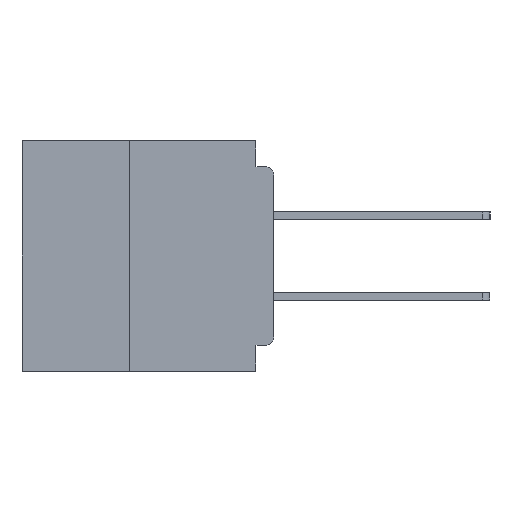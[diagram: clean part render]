
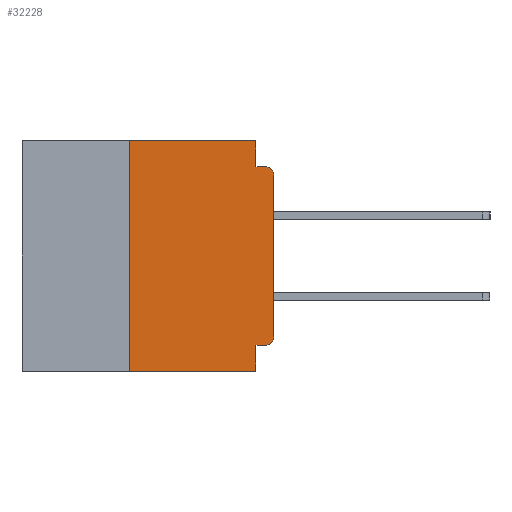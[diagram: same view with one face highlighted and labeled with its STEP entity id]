
A CAD part, left-side view. The second image highlights one B-rep face of the part: STEP entity #32228.
In plain terms, the highlighted planar face has unit normal (-1, 0, 0).
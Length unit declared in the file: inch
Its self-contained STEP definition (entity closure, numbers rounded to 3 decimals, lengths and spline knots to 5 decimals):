
#63 = CARTESIAN_POINT ( 'NONE',  ( 0., 0.031, -0.4 ) ) ;
#301 = FACE_OUTER_BOUND ( 'NONE', #5033, .T. ) ;
#354 = DIRECTION ( 'NONE',  ( 0., 0., -1. ) ) ;
#1073 = EDGE_CURVE ( 'NONE', #8097, #22778, #32696, .T. ) ;
#1078 = CARTESIAN_POINT ( 'NONE',  ( 0., 0.25, 0. ) ) ;
#1639 = LINE ( 'NONE', #37122, #17324 ) ;
#2381 = EDGE_CURVE ( 'NONE', #8097, #33023, #16201, .T. ) ;
#3934 = ORIENTED_EDGE ( 'NONE', *, *, #2381, .T. ) ;
#4353 = EDGE_CURVE ( 'NONE', #19786, #31630, #17419, .T. ) ;
#4840 = VERTEX_POINT ( 'NONE', #6198 ) ;
#4859 = CARTESIAN_POINT ( 'NONE',  ( 0., 0.031, 0. ) ) ;
#5033 = EDGE_LOOP ( 'NONE', ( #5572, #15043, #29890, #26032, #13446, #22626, #3934, #21858, #25732, #12016 ) ) ;
#5572 = ORIENTED_EDGE ( 'NONE', *, *, #6417, .T. ) ;
#5664 = VERTEX_POINT ( 'NONE', #15460 ) ;
#6160 = VECTOR ( 'NONE', #27031, 39.37008 ) ;
#6183 = CARTESIAN_POINT ( 'NONE',  ( 0., 0.015, -0.355 ) ) ;
#6198 = CARTESIAN_POINT ( 'NONE',  ( 0., 0., -0.34 ) ) ;
#6417 = EDGE_CURVE ( 'NONE', #4840, #19786, #29302, .T. ) ;
#8097 = VERTEX_POINT ( 'NONE', #29128 ) ;
#8337 = CARTESIAN_POINT ( 'NONE',  ( 0., 0., -0.045 ) ) ;
#9263 = VECTOR ( 'NONE', #20556, 39.37008 ) ;
#10635 = AXIS2_PLACEMENT_3D ( 'NONE', #28412, #11251, #31383 ) ;
#10794 = DIRECTION ( 'NONE',  ( 0., 0., -1. ) ) ;
#11016 = CARTESIAN_POINT ( 'NONE',  ( 0., 0.031, 0. ) ) ;
#11251 = DIRECTION ( 'NONE',  ( 1., 0., 0. ) ) ;
#11285 = VECTOR ( 'NONE', #16292, 39.37008 ) ;
#12016 = ORIENTED_EDGE ( 'NONE', *, *, #26692, .T. ) ;
#13446 = ORIENTED_EDGE ( 'NONE', *, *, #28144, .F. ) ;
#14056 = PLANE ( 'NONE',  #10635 ) ;
#14420 = LINE ( 'NONE', #8337, #15321 ) ;
#14427 = VECTOR ( 'NONE', #10794, 39.37008 ) ;
#14784 = EDGE_CURVE ( 'NONE', #24814, #5664, #37004, .T. ) ;
#15043 = ORIENTED_EDGE ( 'NONE', *, *, #4353, .T. ) ;
#15321 = VECTOR ( 'NONE', #34233, 39.37008 ) ;
#15460 = CARTESIAN_POINT ( 'NONE',  ( 0., 0.031, -0.045 ) ) ;
#15681 = CARTESIAN_POINT ( 'NONE',  ( 0., 0., -0.06 ) ) ;
#16118 = AXIS2_PLACEMENT_3D ( 'NONE', #17926, #17888, #17855 ) ;
#16201 = LINE ( 'NONE', #20604, #9263 ) ;
#16292 = DIRECTION ( 'NONE',  ( 0., -1., 0. ) ) ;
#17324 = VECTOR ( 'NONE', #20376, 39.37008 ) ;
#17419 = CIRCLE ( 'NONE', #16118, 0.015 ) ;
#17543 = CARTESIAN_POINT ( 'NONE',  ( 0., 0.031, -0.355 ) ) ;
#17855 = DIRECTION ( 'NONE',  ( 0., 0., -1. ) ) ;
#17888 = DIRECTION ( 'NONE',  ( -1., 0., 0. ) ) ;
#17926 = CARTESIAN_POINT ( 'NONE',  ( 0., 0.015, -0.06 ) ) ;
#18024 = DIRECTION ( 'NONE',  ( -1., 0., 0. ) ) ;
#19013 = EDGE_CURVE ( 'NONE', #5664, #31630, #14420, .T. ) ;
#19786 = VERTEX_POINT ( 'NONE', #15681 ) ;
#20376 = DIRECTION ( 'NONE',  ( 0., 1., 0. ) ) ;
#20381 = DIRECTION ( 'NONE',  ( 0., 0., 1. ) ) ;
#20556 = DIRECTION ( 'NONE',  ( 0., -1., 0. ) ) ;
#20604 = CARTESIAN_POINT ( 'NONE',  ( 0., 0.437, -0.4 ) ) ;
#21509 = LINE ( 'NONE', #33501, #35559 ) ;
#21858 = ORIENTED_EDGE ( 'NONE', *, *, #31597, .F. ) ;
#21936 = EDGE_CURVE ( 'NONE', #32441, #28718, #1639, .T. ) ;
#22626 = ORIENTED_EDGE ( 'NONE', *, *, #1073, .F. ) ;
#22778 = VERTEX_POINT ( 'NONE', #1078 ) ;
#24814 = VERTEX_POINT ( 'NONE', #11016 ) ;
#25731 = CARTESIAN_POINT ( 'NONE',  ( 0., 0.015, -0.045 ) ) ;
#25732 = ORIENTED_EDGE ( 'NONE', *, *, #21936, .F. ) ;
#25773 = LINE ( 'NONE', #36072, #11285 ) ;
#26032 = ORIENTED_EDGE ( 'NONE', *, *, #14784, .F. ) ;
#26044 = VECTOR ( 'NONE', #20381, 39.37008 ) ;
#26692 = EDGE_CURVE ( 'NONE', #32441, #4840, #26823, .T. ) ;
#26823 = CIRCLE ( 'NONE', #26956, 0.015 ) ;
#26956 = AXIS2_PLACEMENT_3D ( 'NONE', #34967, #18024, #354 ) ;
#27004 = CARTESIAN_POINT ( 'NONE',  ( 0., 0., 0. ) ) ;
#27031 = DIRECTION ( 'NONE',  ( 0., 0., 1. ) ) ;
#28144 = EDGE_CURVE ( 'NONE', #22778, #24814, #25773, .T. ) ;
#28412 = CARTESIAN_POINT ( 'NONE',  ( 0., 0.437, 0. ) ) ;
#28718 = VERTEX_POINT ( 'NONE', #17543 ) ;
#29128 = CARTESIAN_POINT ( 'NONE',  ( 0., 0.25, -0.4 ) ) ;
#29302 = LINE ( 'NONE', #27004, #6160 ) ;
#29890 = ORIENTED_EDGE ( 'NONE', *, *, #19013, .F. ) ;
#31383 = DIRECTION ( 'NONE',  ( 0., 0., -1. ) ) ;
#31597 = EDGE_CURVE ( 'NONE', #28718, #33023, #21509, .T. ) ;
#31630 = VERTEX_POINT ( 'NONE', #25731 ) ;
#31763 = CARTESIAN_POINT ( 'NONE',  ( 0., 0.25, -0.4 ) ) ;
#32228 = ADVANCED_FACE ( 'NONE', ( #301 ), #14056, .F. ) ;
#32441 = VERTEX_POINT ( 'NONE', #6183 ) ;
#32696 = LINE ( 'NONE', #31763, #26044 ) ;
#33023 = VERTEX_POINT ( 'NONE', #63 ) ;
#33501 = CARTESIAN_POINT ( 'NONE',  ( 0., 0.031, -0.4 ) ) ;
#34233 = DIRECTION ( 'NONE',  ( 0., -1., 0. ) ) ;
#34967 = CARTESIAN_POINT ( 'NONE',  ( 0., 0.015, -0.34 ) ) ;
#35559 = VECTOR ( 'NONE', #36215, 39.37008 ) ;
#36072 = CARTESIAN_POINT ( 'NONE',  ( 0., 0.437, 0. ) ) ;
#36215 = DIRECTION ( 'NONE',  ( 0., 0., -1. ) ) ;
#37004 = LINE ( 'NONE', #4859, #14427 ) ;
#37122 = CARTESIAN_POINT ( 'NONE',  ( 0., 0., -0.355 ) ) ;
